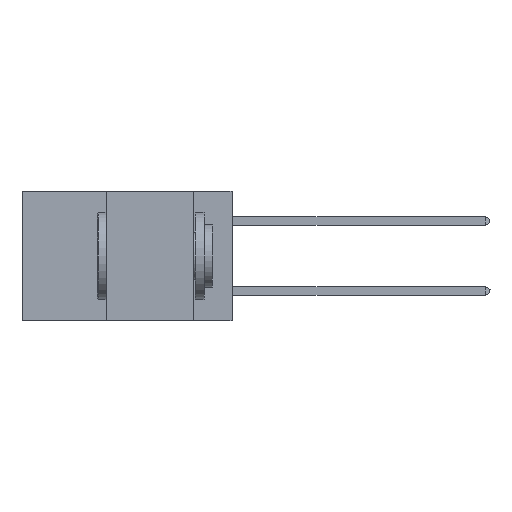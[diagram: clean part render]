
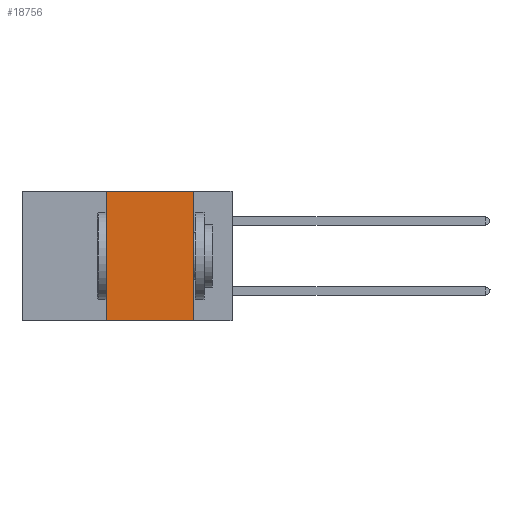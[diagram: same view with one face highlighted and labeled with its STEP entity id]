
A CAD part, left-side view. The second image highlights one B-rep face of the part: STEP entity #18756.
In plain terms, the highlighted planar face has unit normal (-1, 0, 0).
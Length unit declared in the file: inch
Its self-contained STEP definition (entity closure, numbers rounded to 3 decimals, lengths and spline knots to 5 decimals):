
#119 = CARTESIAN_POINT ( 'NONE',  ( 0., 0.11, 0. ) ) ;
#1577 = DIRECTION ( 'NONE',  ( 0., -1., 0. ) ) ;
#1841 = VERTEX_POINT ( 'NONE', #119 ) ;
#3235 = FACE_OUTER_BOUND ( 'NONE', #7864, .T. ) ;
#4312 = LINE ( 'NONE', #22549, #15722 ) ;
#4732 = CARTESIAN_POINT ( 'NONE',  ( 0., 0.6, 0. ) ) ;
#5192 = LINE ( 'NONE', #26398, #16566 ) ;
#5630 = VERTEX_POINT ( 'NONE', #12244 ) ;
#6395 = CARTESIAN_POINT ( 'NONE',  ( 0., 0.36, 0. ) ) ;
#7063 = DIRECTION ( 'NONE',  ( 0., 0., -1. ) ) ;
#7864 = EDGE_LOOP ( 'NONE', ( #27536, #17875, #14729, #15436 ) ) ;
#7904 = EDGE_CURVE ( 'NONE', #5630, #27679, #19849, .T. ) ;
#7905 = VECTOR ( 'NONE', #11139, 39.37008 ) ;
#8855 = CARTESIAN_POINT ( 'NONE',  ( 0., 0.6, -0.37 ) ) ;
#9279 = CARTESIAN_POINT ( 'NONE',  ( 0., 0.11, 0. ) ) ;
#10619 = CARTESIAN_POINT ( 'NONE',  ( 0., 0.11, -0.37 ) ) ;
#11139 = DIRECTION ( 'NONE',  ( 0., -1., 0. ) ) ;
#11440 = DIRECTION ( 'NONE',  ( 0., 0., 1. ) ) ;
#11566 = DIRECTION ( 'NONE',  ( 0., 0., -1. ) ) ;
#12244 = CARTESIAN_POINT ( 'NONE',  ( 0., 0.36, -0.37 ) ) ;
#12876 = EDGE_CURVE ( 'NONE', #1841, #27679, #29006, .T. ) ;
#14729 = ORIENTED_EDGE ( 'NONE', *, *, #19385, .F. ) ;
#15436 = ORIENTED_EDGE ( 'NONE', *, *, #7904, .T. ) ;
#15722 = VECTOR ( 'NONE', #11440, 39.37008 ) ;
#16544 = EDGE_CURVE ( 'NONE', #18056, #1841, #5192, .T. ) ;
#16566 = VECTOR ( 'NONE', #1577, 39.37008 ) ;
#16576 = VECTOR ( 'NONE', #11566, 39.37008 ) ;
#17875 = ORIENTED_EDGE ( 'NONE', *, *, #16544, .F. ) ;
#18056 = VERTEX_POINT ( 'NONE', #6395 ) ;
#18756 = ADVANCED_FACE ( 'NONE', ( #3235 ), #27113, .F. ) ;
#19385 = EDGE_CURVE ( 'NONE', #5630, #18056, #4312, .T. ) ;
#19849 = LINE ( 'NONE', #8855, #7905 ) ;
#20526 = DIRECTION ( 'NONE',  ( 1., 0., 0. ) ) ;
#22549 = CARTESIAN_POINT ( 'NONE',  ( 0., 0.36, 0. ) ) ;
#25370 = AXIS2_PLACEMENT_3D ( 'NONE', #4732, #20526, #7063 ) ;
#26398 = CARTESIAN_POINT ( 'NONE',  ( 0., 0.6, 0. ) ) ;
#27113 = PLANE ( 'NONE',  #25370 ) ;
#27536 = ORIENTED_EDGE ( 'NONE', *, *, #12876, .F. ) ;
#27679 = VERTEX_POINT ( 'NONE', #10619 ) ;
#29006 = LINE ( 'NONE', #9279, #16576 ) ;
